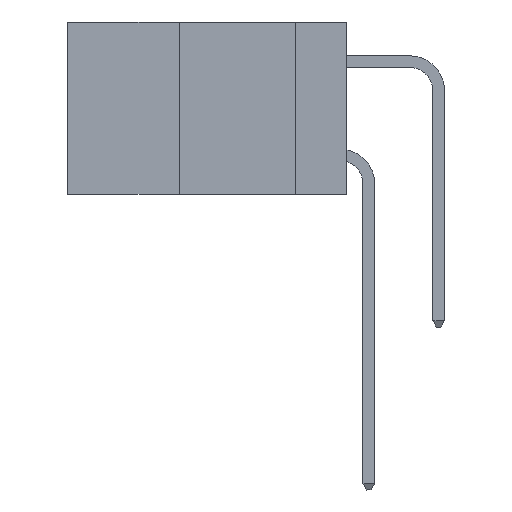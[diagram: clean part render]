
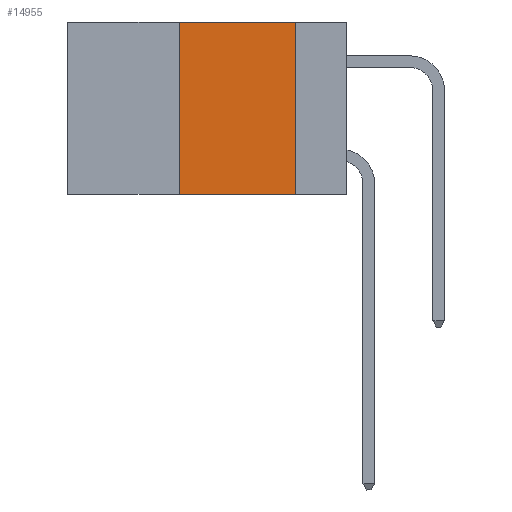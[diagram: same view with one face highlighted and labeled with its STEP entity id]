
A CAD part, left-side view. The second image highlights one B-rep face of the part: STEP entity #14955.
In plain terms, the highlighted planar face has unit normal (-1, 0, 0).
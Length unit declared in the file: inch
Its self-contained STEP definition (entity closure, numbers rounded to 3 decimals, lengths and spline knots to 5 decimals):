
#273 = ORIENTED_EDGE ( 'NONE', *, *, #5212, .F. ) ;
#547 = VERTEX_POINT ( 'NONE', #12572 ) ;
#609 = VECTOR ( 'NONE', #15010, 39.37008 ) ;
#861 = ORIENTED_EDGE ( 'NONE', *, *, #4613, .F. ) ;
#1901 = PLANE ( 'NONE',  #7591 ) ;
#1998 = LINE ( 'NONE', #11249, #14064 ) ;
#2514 = VERTEX_POINT ( 'NONE', #8684 ) ;
#2762 = DIRECTION ( 'NONE',  ( 0., 0., 1. ) ) ;
#3190 = DIRECTION ( 'NONE',  ( 0., 0., -1. ) ) ;
#3294 = CARTESIAN_POINT ( 'NONE',  ( 0., 0.11, 0. ) ) ;
#3455 = CARTESIAN_POINT ( 'NONE',  ( 0., 0.36, -0.37 ) ) ;
#3990 = CARTESIAN_POINT ( 'NONE',  ( 0., 0.6, -0.37 ) ) ;
#4493 = VERTEX_POINT ( 'NONE', #3294 ) ;
#4613 = EDGE_CURVE ( 'NONE', #2514, #4493, #10499, .T. ) ;
#4849 = ORIENTED_EDGE ( 'NONE', *, *, #5274, .F. ) ;
#5150 = CARTESIAN_POINT ( 'NONE',  ( 0., 0.11, 0. ) ) ;
#5212 = EDGE_CURVE ( 'NONE', #4493, #547, #7327, .T. ) ;
#5243 = EDGE_CURVE ( 'NONE', #5925, #547, #12657, .T. ) ;
#5270 = DIRECTION ( 'NONE',  ( 0., -1., 0. ) ) ;
#5274 = EDGE_CURVE ( 'NONE', #5925, #2514, #1998, .T. ) ;
#5651 = ORIENTED_EDGE ( 'NONE', *, *, #5243, .T. ) ;
#5925 = VERTEX_POINT ( 'NONE', #3455 ) ;
#6098 = FACE_OUTER_BOUND ( 'NONE', #6602, .T. ) ;
#6425 = DIRECTION ( 'NONE',  ( 0., 0., -1. ) ) ;
#6602 = EDGE_LOOP ( 'NONE', ( #273, #861, #4849, #5651 ) ) ;
#7327 = LINE ( 'NONE', #5150, #10083 ) ;
#7591 = AXIS2_PLACEMENT_3D ( 'NONE', #13634, #10494, #3190 ) ;
#8684 = CARTESIAN_POINT ( 'NONE',  ( 0., 0.36, 0. ) ) ;
#10083 = VECTOR ( 'NONE', #6425, 39.37008 ) ;
#10494 = DIRECTION ( 'NONE',  ( 1., 0., 0. ) ) ;
#10499 = LINE ( 'NONE', #13957, #609 ) ;
#11249 = CARTESIAN_POINT ( 'NONE',  ( 0., 0.36, 0. ) ) ;
#12572 = CARTESIAN_POINT ( 'NONE',  ( 0., 0.11, -0.37 ) ) ;
#12657 = LINE ( 'NONE', #3990, #14729 ) ;
#13634 = CARTESIAN_POINT ( 'NONE',  ( 0., 0.6, 0. ) ) ;
#13957 = CARTESIAN_POINT ( 'NONE',  ( 0., 0.6, 0. ) ) ;
#14064 = VECTOR ( 'NONE', #2762, 39.37008 ) ;
#14729 = VECTOR ( 'NONE', #5270, 39.37008 ) ;
#14955 = ADVANCED_FACE ( 'NONE', ( #6098 ), #1901, .F. ) ;
#15010 = DIRECTION ( 'NONE',  ( 0., -1., 0. ) ) ;
